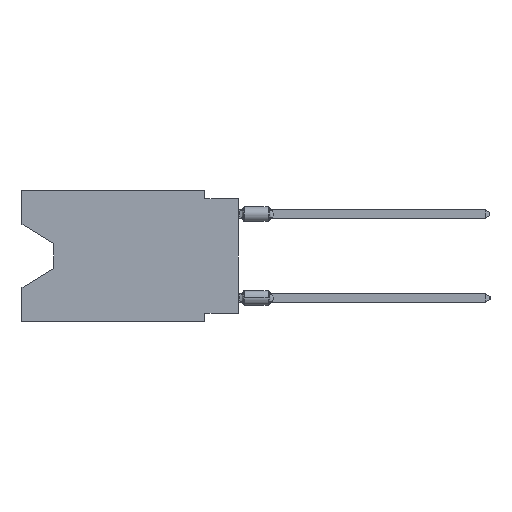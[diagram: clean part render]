
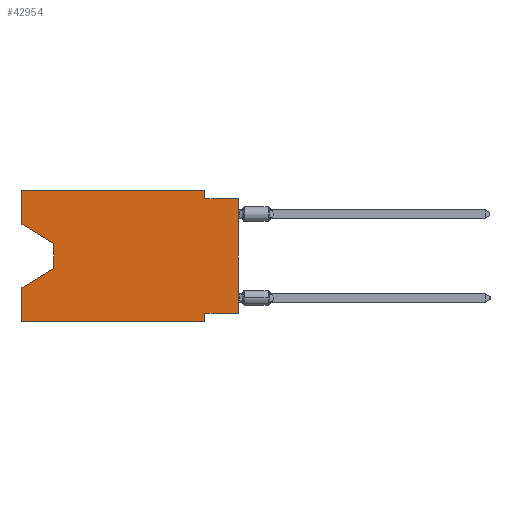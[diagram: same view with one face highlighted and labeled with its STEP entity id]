
A CAD part, left-side view. The second image highlights one B-rep face of the part: STEP entity #42954.
In plain terms, the highlighted planar face has unit normal (-1, 0, 0).
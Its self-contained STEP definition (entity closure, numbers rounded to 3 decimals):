
#239 = LINE ( 'NONE', #20796, #1478 ) ;
#254 = VECTOR ( 'NONE', #21050, 1000. ) ;
#992 = VECTOR ( 'NONE', #3427, 1000. ) ;
#1158 = EDGE_CURVE ( 'NONE', #6592, #31742, #19383, .T. ) ;
#1247 = LINE ( 'NONE', #4893, #31142 ) ;
#1478 = VECTOR ( 'NONE', #27198, 1000. ) ;
#1631 = VERTEX_POINT ( 'NONE', #41051 ) ;
#2189 = ORIENTED_EDGE ( 'NONE', *, *, #5974, .F. ) ;
#2292 = DIRECTION ( 'NONE',  ( 0., -1., 0. ) ) ;
#2555 = CARTESIAN_POINT ( 'NONE',  ( 0., 2.54, 0. ) ) ;
#2901 = CARTESIAN_POINT ( 'NONE',  ( 0., 13.97, -4.013 ) ) ;
#3114 = ORIENTED_EDGE ( 'NONE', *, *, #32453, .T. ) ;
#3427 = DIRECTION ( 'NONE',  ( 0., 0., 1. ) ) ;
#3759 = CARTESIAN_POINT ( 'NONE',  ( 0., 0., -0.635 ) ) ;
#3919 = EDGE_CURVE ( 'NONE', #31742, #1631, #8811, .T. ) ;
#4893 = CARTESIAN_POINT ( 'NONE',  ( 0., 16.383, 0. ) ) ;
#5054 = LINE ( 'NONE', #8709, #11237 ) ;
#5974 = EDGE_CURVE ( 'NONE', #6001, #25455, #34997, .T. ) ;
#6001 = VERTEX_POINT ( 'NONE', #7308 ) ;
#6592 = VERTEX_POINT ( 'NONE', #37880 ) ;
#7124 = CARTESIAN_POINT ( 'NONE',  ( 0., 0., 0. ) ) ;
#7198 = DIRECTION ( 'NONE',  ( 0., -1., 0. ) ) ;
#7308 = CARTESIAN_POINT ( 'NONE',  ( 0., 16.383, 0. ) ) ;
#7816 = CARTESIAN_POINT ( 'NONE',  ( 0., 16.383, -9.906 ) ) ;
#8496 = ORIENTED_EDGE ( 'NONE', *, *, #25989, .F. ) ;
#8709 = CARTESIAN_POINT ( 'NONE',  ( 0., 16.383, -9.906 ) ) ;
#8811 = LINE ( 'NONE', #13128, #44693 ) ;
#9309 = ORIENTED_EDGE ( 'NONE', *, *, #3919, .T. ) ;
#10732 = EDGE_CURVE ( 'NONE', #28770, #31981, #26304, .T. ) ;
#11237 = VECTOR ( 'NONE', #2292, 1000. ) ;
#11739 = DIRECTION ( 'NONE',  ( 0., 0., 1. ) ) ;
#13055 = PLANE ( 'NONE',  #15242 ) ;
#13128 = CARTESIAN_POINT ( 'NONE',  ( 0., 13.97, -4.013 ) ) ;
#14221 = VECTOR ( 'NONE', #40006, 1000. ) ;
#15242 = AXIS2_PLACEMENT_3D ( 'NONE', #23548, #33870, #41430 ) ;
#15515 = CARTESIAN_POINT ( 'NONE',  ( 0., 16.383, -2.546 ) ) ;
#16266 = CARTESIAN_POINT ( 'NONE',  ( 0., 16.383, -7.36 ) ) ;
#16290 = CARTESIAN_POINT ( 'NONE',  ( 0., 0., -9.271 ) ) ;
#16687 = CARTESIAN_POINT ( 'NONE',  ( 0., 16.383, 0. ) ) ;
#18270 = LINE ( 'NONE', #39113, #25259 ) ;
#19019 = EDGE_CURVE ( 'NONE', #6592, #6001, #1247, .T. ) ;
#19383 = LINE ( 'NONE', #15515, #14221 ) ;
#20434 = VERTEX_POINT ( 'NONE', #16290 ) ;
#20455 = VECTOR ( 'NONE', #32861, 1000. ) ;
#20782 = LINE ( 'NONE', #34766, #992 ) ;
#20796 = CARTESIAN_POINT ( 'NONE',  ( 0., 2.54, 0. ) ) ;
#20854 = EDGE_CURVE ( 'NONE', #25455, #21248, #239, .T. ) ;
#21050 = DIRECTION ( 'NONE',  ( 0., 0., 1. ) ) ;
#21248 = VERTEX_POINT ( 'NONE', #40903 ) ;
#22987 = VECTOR ( 'NONE', #37527, 1000. ) ;
#23404 = DIRECTION ( 'NONE',  ( 0., 0., -1. ) ) ;
#23548 = CARTESIAN_POINT ( 'NONE',  ( 0., 16.383, 0. ) ) ;
#24079 = ORIENTED_EDGE ( 'NONE', *, *, #19019, .F. ) ;
#25259 = VECTOR ( 'NONE', #31780, 1000. ) ;
#25455 = VERTEX_POINT ( 'NONE', #2555 ) ;
#25524 = LINE ( 'NONE', #43180, #20455 ) ;
#25989 = EDGE_CURVE ( 'NONE', #20434, #28770, #25524, .T. ) ;
#26304 = LINE ( 'NONE', #40072, #22987 ) ;
#26856 = ORIENTED_EDGE ( 'NONE', *, *, #10732, .F. ) ;
#26997 = FACE_OUTER_BOUND ( 'NONE', #39385, .T. ) ;
#27198 = DIRECTION ( 'NONE',  ( 0., 0., -1. ) ) ;
#27272 = EDGE_CURVE ( 'NONE', #40648, #30934, #20782, .T. ) ;
#28077 = EDGE_CURVE ( 'NONE', #21248, #37105, #41735, .T. ) ;
#28770 = VERTEX_POINT ( 'NONE', #40677 ) ;
#30934 = VERTEX_POINT ( 'NONE', #16266 ) ;
#31114 = EDGE_CURVE ( 'NONE', #20434, #37105, #38460, .T. ) ;
#31142 = VECTOR ( 'NONE', #11739, 1000. ) ;
#31247 = CARTESIAN_POINT ( 'NONE',  ( 0., 2.54, -9.906 ) ) ;
#31538 = DIRECTION ( 'NONE',  ( 0., -1., 0. ) ) ;
#31742 = VERTEX_POINT ( 'NONE', #2901 ) ;
#31780 = DIRECTION ( 'NONE',  ( 0., 0.855, -0.519 ) ) ;
#31981 = VERTEX_POINT ( 'NONE', #31247 ) ;
#32223 = ORIENTED_EDGE ( 'NONE', *, *, #36858, .T. ) ;
#32453 = EDGE_CURVE ( 'NONE', #40648, #31981, #5054, .T. ) ;
#32696 = CARTESIAN_POINT ( 'NONE',  ( 0., 0., -0.635 ) ) ;
#32861 = DIRECTION ( 'NONE',  ( 0., 1., 0. ) ) ;
#33870 = DIRECTION ( 'NONE',  ( 1., 0., 0. ) ) ;
#34766 = CARTESIAN_POINT ( 'NONE',  ( 0., 16.383, 0. ) ) ;
#34997 = LINE ( 'NONE', #16687, #39701 ) ;
#36858 = EDGE_CURVE ( 'NONE', #1631, #30934, #18270, .T. ) ;
#37105 = VERTEX_POINT ( 'NONE', #32696 ) ;
#37527 = DIRECTION ( 'NONE',  ( 0., 0., -1. ) ) ;
#37880 = CARTESIAN_POINT ( 'NONE',  ( 0., 16.383, -2.546 ) ) ;
#38460 = LINE ( 'NONE', #7124, #254 ) ;
#38885 = VECTOR ( 'NONE', #7198, 1000. ) ;
#39113 = CARTESIAN_POINT ( 'NONE',  ( 0., 13.97, -5.893 ) ) ;
#39385 = EDGE_LOOP ( 'NONE', ( #42811, #9309, #32223, #41797, #3114, #26856, #8496, #42887, #43470, #45226, #2189, #24079 ) ) ;
#39701 = VECTOR ( 'NONE', #31538, 1000. ) ;
#40006 = DIRECTION ( 'NONE',  ( 0., -0.855, -0.519 ) ) ;
#40072 = CARTESIAN_POINT ( 'NONE',  ( 0., 2.54, -9.906 ) ) ;
#40648 = VERTEX_POINT ( 'NONE', #7816 ) ;
#40677 = CARTESIAN_POINT ( 'NONE',  ( 0., 2.54, -9.271 ) ) ;
#40903 = CARTESIAN_POINT ( 'NONE',  ( 0., 2.54, -0.635 ) ) ;
#41051 = CARTESIAN_POINT ( 'NONE',  ( 0., 13.97, -5.893 ) ) ;
#41430 = DIRECTION ( 'NONE',  ( 0., 0., -1. ) ) ;
#41735 = LINE ( 'NONE', #3759, #38885 ) ;
#41797 = ORIENTED_EDGE ( 'NONE', *, *, #27272, .F. ) ;
#42811 = ORIENTED_EDGE ( 'NONE', *, *, #1158, .T. ) ;
#42887 = ORIENTED_EDGE ( 'NONE', *, *, #31114, .T. ) ;
#42954 = ADVANCED_FACE ( 'NONE', ( #26997 ), #13055, .F. ) ;
#43180 = CARTESIAN_POINT ( 'NONE',  ( 0., 0., -9.271 ) ) ;
#43470 = ORIENTED_EDGE ( 'NONE', *, *, #28077, .F. ) ;
#44693 = VECTOR ( 'NONE', #23404, 1000. ) ;
#45226 = ORIENTED_EDGE ( 'NONE', *, *, #20854, .F. ) ;
